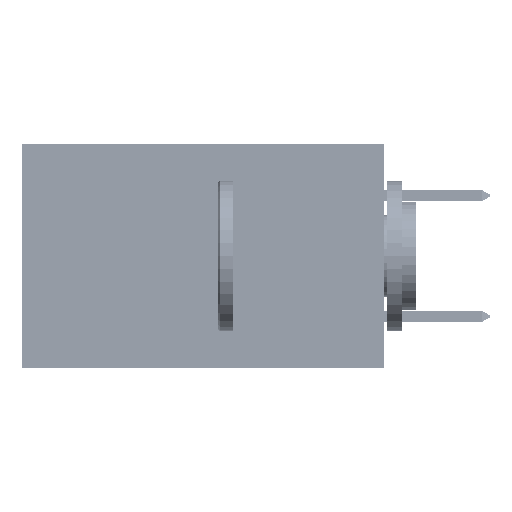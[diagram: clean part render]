
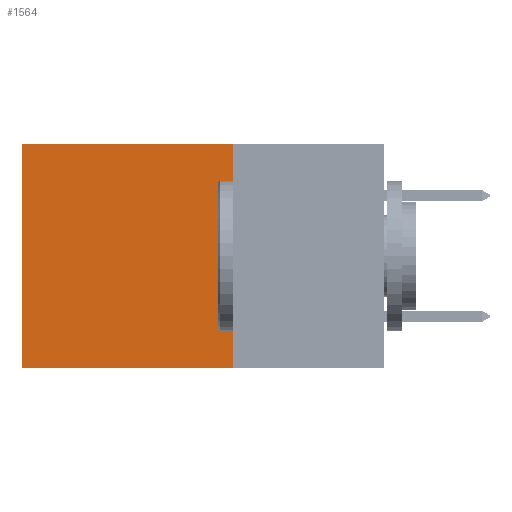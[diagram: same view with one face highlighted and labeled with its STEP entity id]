
A CAD part, left-side view. The second image highlights one B-rep face of the part: STEP entity #1564.
In plain terms, the highlighted planar face has unit normal (-1, 0, 0).
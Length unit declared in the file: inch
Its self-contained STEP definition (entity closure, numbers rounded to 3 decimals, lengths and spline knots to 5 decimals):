
#1384 = EDGE_CURVE ( 'NONE', #26989, #26131, #26001, .T. ) ;
#1564 = ADVANCED_FACE ( 'NONE', ( #48839 ), #40473, .F. ) ;
#4376 = LINE ( 'NONE', #17327, #45289 ) ;
#7370 = ORIENTED_EDGE ( 'NONE', *, *, #48537, .T. ) ;
#7743 = VECTOR ( 'NONE', #22936, 39.37008 ) ;
#8313 = LINE ( 'NONE', #35070, #37527 ) ;
#8912 = EDGE_CURVE ( 'NONE', #20660, #26989, #4376, .T. ) ;
#14314 = CARTESIAN_POINT ( 'NONE',  ( 0.2875, 0.25, 0. ) ) ;
#15277 = DIRECTION ( 'NONE',  ( 0., 0., -1. ) ) ;
#15499 = DIRECTION ( 'NONE',  ( 0., 1., 0. ) ) ;
#15628 = ORIENTED_EDGE ( 'NONE', *, *, #8912, .F. ) ;
#16060 = AXIS2_PLACEMENT_3D ( 'NONE', #16697, #44397, #20694 ) ;
#16697 = CARTESIAN_POINT ( 'NONE',  ( 0.2875, 0.25, 0. ) ) ;
#17327 = CARTESIAN_POINT ( 'NONE',  ( 0.2875, 0.25, 0. ) ) ;
#17331 = CARTESIAN_POINT ( 'NONE',  ( 0.2875, 0.6, -0.37 ) ) ;
#19324 = CARTESIAN_POINT ( 'NONE',  ( 0.2875, 0.25, -0.37 ) ) ;
#20660 = VERTEX_POINT ( 'NONE', #14314 ) ;
#20694 = DIRECTION ( 'NONE',  ( 0., 0., -1. ) ) ;
#22936 = DIRECTION ( 'NONE',  ( 0., 1., 0. ) ) ;
#25183 = CARTESIAN_POINT ( 'NONE',  ( 0.2875, 0.6, 0. ) ) ;
#26001 = LINE ( 'NONE', #19324, #27234 ) ;
#26131 = VERTEX_POINT ( 'NONE', #17331 ) ;
#26673 = ORIENTED_EDGE ( 'NONE', *, *, #1384, .F. ) ;
#26989 = VERTEX_POINT ( 'NONE', #34601 ) ;
#27234 = VECTOR ( 'NONE', #15499, 39.37008 ) ;
#27258 = ORIENTED_EDGE ( 'NONE', *, *, #33919, .T. ) ;
#30209 = LINE ( 'NONE', #34772, #7743 ) ;
#33321 = DIRECTION ( 'NONE',  ( 0., 0., -1. ) ) ;
#33386 = EDGE_LOOP ( 'NONE', ( #7370, #26673, #15628, #27258 ) ) ;
#33919 = EDGE_CURVE ( 'NONE', #20660, #46350, #30209, .T. ) ;
#34601 = CARTESIAN_POINT ( 'NONE',  ( 0.2875, 0.25, -0.37 ) ) ;
#34772 = CARTESIAN_POINT ( 'NONE',  ( 0.2875, 0.25, 0. ) ) ;
#35070 = CARTESIAN_POINT ( 'NONE',  ( 0.2875, 0.6, 0. ) ) ;
#37527 = VECTOR ( 'NONE', #15277, 39.37008 ) ;
#40473 = PLANE ( 'NONE',  #16060 ) ;
#44397 = DIRECTION ( 'NONE',  ( 1., 0., 0. ) ) ;
#45289 = VECTOR ( 'NONE', #33321, 39.37008 ) ;
#46350 = VERTEX_POINT ( 'NONE', #25183 ) ;
#48537 = EDGE_CURVE ( 'NONE', #46350, #26131, #8313, .T. ) ;
#48839 = FACE_OUTER_BOUND ( 'NONE', #33386, .T. ) ;
